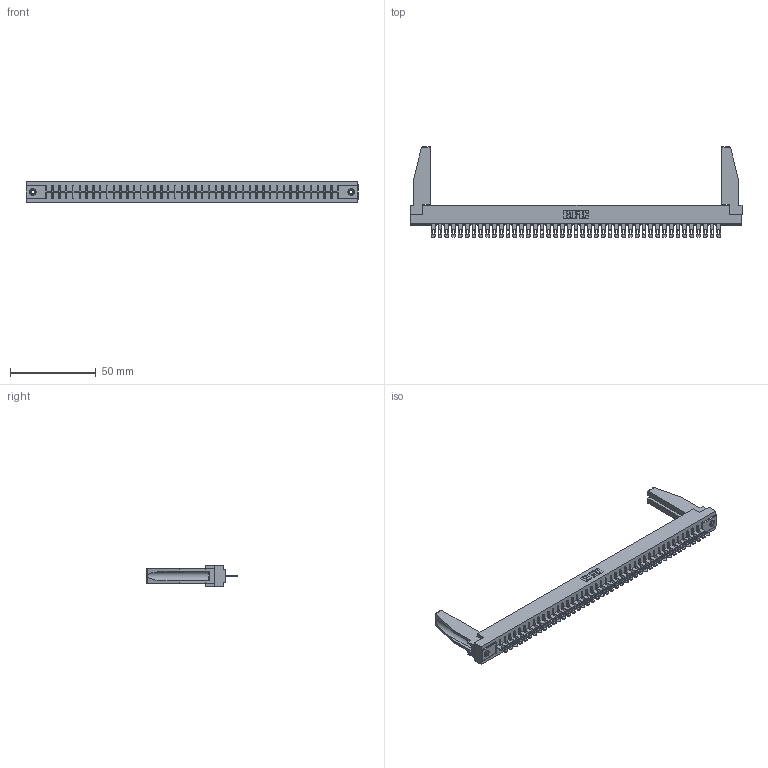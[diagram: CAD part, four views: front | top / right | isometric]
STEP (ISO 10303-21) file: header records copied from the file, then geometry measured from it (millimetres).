
FILE_DESCRIPTION (( 'STEP AP203' ), '1' );
FILE_NAME ('306-043-400-178.STEP', '2020-09-22T13:22:09', ( '' ), ( '' ), 'SwSTEP 2.0', 'SolidWorks 2020', '' );
FILE_SCHEMA (( 'CONFIG_CONTROL_DESIGN' ));
Length unit declared in the file: inch
Products named in the file (5): 306-290-001_100; 306-043-400-178; 345-250-001_345-250-001-102; 307-220-078; 306 Part_.156 Dia
Assembly tree (48 placements, depth 2):
  306-043-400-178
    306 Part_.156 Dia
    306-290-001_100  x43
    345-250-001_345-250-001-102  x2
    307-220-078  x2
Bounding box: 193.4 x 52.91 x 12.7 mm (x, y, z)
Volume: 25528.7 mm3; surface area: 26704.9 mm2
Topology: 48 solids, 48 shells, 3514 faces, 9891 edges, 6354 vertices
Faces by surface type: plane 2302, cylinder 1024, sphere 172, cone 12, torus 4
Entity records: 42573 total; most frequent: CARTESIAN_POINT 7150, ORIENTED_EDGE 7048, DIRECTION 7002, EDGE_CURVE 3524, VECTOR 2758, LINE 2758, VERTEX_POINT 2228, AXIS2_PLACEMENT_3D 2122
